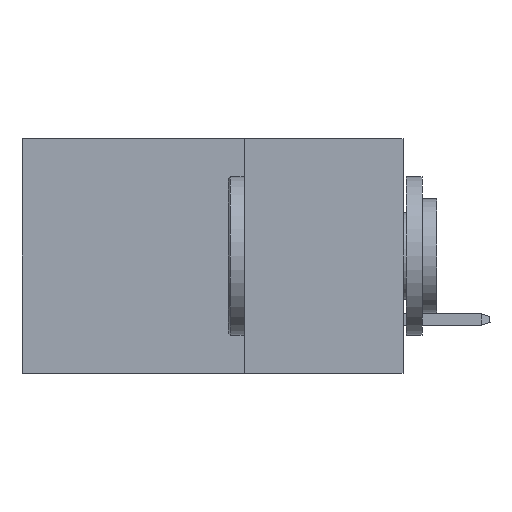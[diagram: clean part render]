
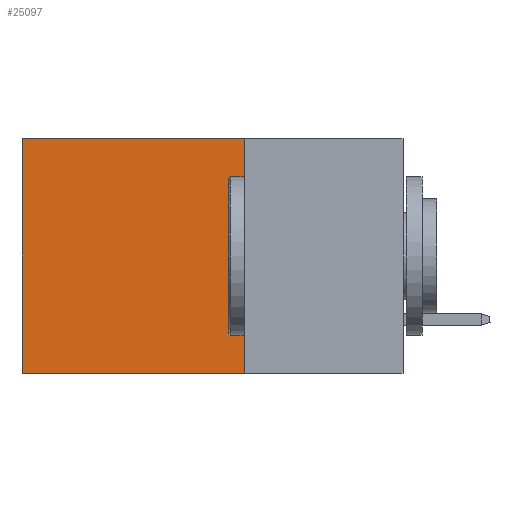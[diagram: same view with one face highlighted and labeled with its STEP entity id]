
A CAD part, left-side view. The second image highlights one B-rep face of the part: STEP entity #25097.
In plain terms, the highlighted planar face has unit normal (-1, 0, 0).
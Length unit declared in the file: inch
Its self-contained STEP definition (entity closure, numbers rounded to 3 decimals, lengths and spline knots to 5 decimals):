
#151 = VERTEX_POINT ( 'NONE', #9392 ) ;
#1420 = CARTESIAN_POINT ( 'NONE',  ( 0.2875, 0.25, -0.37 ) ) ;
#1653 = LINE ( 'NONE', #9354, #17940 ) ;
#1946 = ORIENTED_EDGE ( 'NONE', *, *, #28051, .F. ) ;
#2205 = LINE ( 'NONE', #9742, #18983 ) ;
#4707 = CARTESIAN_POINT ( 'NONE',  ( 0.2875, 0.6, -0.37 ) ) ;
#5510 = EDGE_CURVE ( 'NONE', #25969, #151, #7740, .T. ) ;
#5605 = DIRECTION ( 'NONE',  ( 0., 1., 0. ) ) ;
#6519 = LINE ( 'NONE', #1420, #19970 ) ;
#7740 = LINE ( 'NONE', #10343, #28106 ) ;
#8780 = EDGE_LOOP ( 'NONE', ( #27495, #1946, #22256, #17243 ) ) ;
#8843 = CARTESIAN_POINT ( 'NONE',  ( 0.2875, 0.25, 0. ) ) ;
#9030 = DIRECTION ( 'NONE',  ( 0., 0., -1. ) ) ;
#9353 = CARTESIAN_POINT ( 'NONE',  ( 0.2875, 0.25, 0. ) ) ;
#9354 = CARTESIAN_POINT ( 'NONE',  ( 0.2875, 0.25, 0. ) ) ;
#9390 = VERTEX_POINT ( 'NONE', #12968 ) ;
#9392 = CARTESIAN_POINT ( 'NONE',  ( 0.2875, 0.6, 0. ) ) ;
#9742 = CARTESIAN_POINT ( 'NONE',  ( 0.2875, 0.6, 0. ) ) ;
#10343 = CARTESIAN_POINT ( 'NONE',  ( 0.2875, 0.25, 0. ) ) ;
#11471 = PLANE ( 'NONE',  #26607 ) ;
#12968 = CARTESIAN_POINT ( 'NONE',  ( 0.2875, 0.25, -0.37 ) ) ;
#15153 = VERTEX_POINT ( 'NONE', #4707 ) ;
#15572 = EDGE_CURVE ( 'NONE', #151, #15153, #2205, .T. ) ;
#17243 = ORIENTED_EDGE ( 'NONE', *, *, #5510, .T. ) ;
#17940 = VECTOR ( 'NONE', #9030, 39.37008 ) ;
#18682 = FACE_OUTER_BOUND ( 'NONE', #8780, .T. ) ;
#18983 = VECTOR ( 'NONE', #27422, 39.37008 ) ;
#19565 = EDGE_CURVE ( 'NONE', #25969, #9390, #1653, .T. ) ;
#19970 = VECTOR ( 'NONE', #21081, 39.37008 ) ;
#20966 = DIRECTION ( 'NONE',  ( 1., 0., 0. ) ) ;
#21081 = DIRECTION ( 'NONE',  ( 0., 1., 0. ) ) ;
#22256 = ORIENTED_EDGE ( 'NONE', *, *, #19565, .F. ) ;
#25097 = ADVANCED_FACE ( 'NONE', ( #18682 ), #11471, .F. ) ;
#25969 = VERTEX_POINT ( 'NONE', #9353 ) ;
#26607 = AXIS2_PLACEMENT_3D ( 'NONE', #8843, #20966, #31417 ) ;
#27422 = DIRECTION ( 'NONE',  ( 0., 0., -1. ) ) ;
#27495 = ORIENTED_EDGE ( 'NONE', *, *, #15572, .T. ) ;
#28051 = EDGE_CURVE ( 'NONE', #9390, #15153, #6519, .T. ) ;
#28106 = VECTOR ( 'NONE', #5605, 39.37008 ) ;
#31417 = DIRECTION ( 'NONE',  ( 0., 0., -1. ) ) ;
